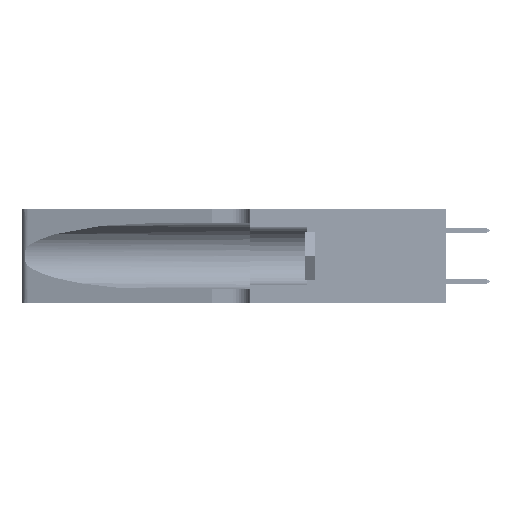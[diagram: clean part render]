
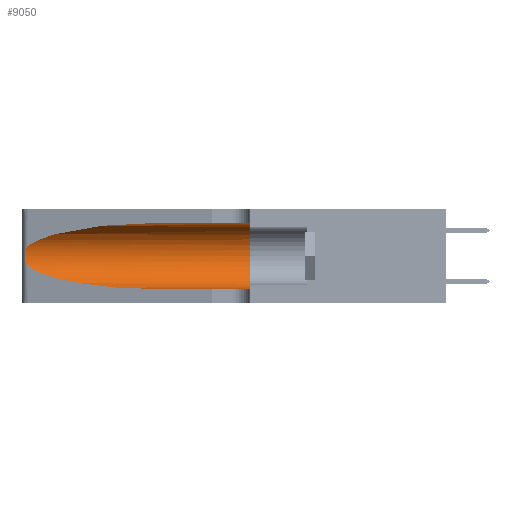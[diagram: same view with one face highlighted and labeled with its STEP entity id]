
A CAD part, left-side view. The second image highlights one B-rep face of the part: STEP entity #9050.
In plain terms, the highlighted cylindrical face has radius 3.308 mm (diameter 6.617 mm), a partial arc.
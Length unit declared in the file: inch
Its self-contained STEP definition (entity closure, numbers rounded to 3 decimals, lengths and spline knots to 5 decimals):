
#23 = VERTEX_POINT ( 'NONE', #31470 ) ;
#273 = CARTESIAN_POINT ( 'NONE',  ( 0.26075, 1.23896, 0.19203 ) ) ;
#2504 = CARTESIAN_POINT ( 'NONE',  ( 0.1305, 1.61858, 0.185 ) ) ;
#2601 = VERTEX_POINT ( 'NONE', #44118 ) ;
#2949 = CARTESIAN_POINT ( 'NONE',  ( 0.1305, 0.35, 0.185 ) ) ;
#3260 = AXIS2_PLACEMENT_3D ( 'NONE', #2504, #6538, #38540 ) ;
#3950 = CARTESIAN_POINT ( 'NONE',  ( 0.25787, 1.23484, 0.2124 ) ) ;
#6538 = DIRECTION ( 'NONE',  ( 0., -1., 0. ) ) ;
#7451 = CYLINDRICAL_SURFACE ( 'NONE', #3260, 0.13025 ) ;
#7989 = CIRCLE ( 'NONE', #35753, 0.13025 ) ;
#8011 = CARTESIAN_POINT ( 'NONE',  ( 0.1305, 1.61858, 0.31525 ) ) ;
#9050 = ADVANCED_FACE ( 'NONE', ( #36763 ), #7451, .F. ) ;
#10402 = DIRECTION ( 'NONE',  ( 0., -1., 0. ) ) ;
#10973 = DIRECTION ( 'NONE',  ( 0., 0., 1. ) ) ;
#11427 = CARTESIAN_POINT ( 'NONE',  ( 0.2373, 1.15595, 0.08982 ) ) ;
#11618 = CARTESIAN_POINT ( 'NONE',  ( 0.25639, 1.23186, 0.15144 ) ) ;
#13715 = EDGE_CURVE ( 'NONE', #27777, #23, #7989, .T. ) ;
#14352 = VERTEX_POINT ( 'NONE', #33731 ) ;
#14677 = CARTESIAN_POINT ( 'NONE',  ( 0.2373, 1.15595, 0.28018 ) ) ;
#16344 = LINE ( 'NONE', #8011, #45632 ) ;
#19237 = CARTESIAN_POINT ( 'NONE',  ( 0.18966, 0.96281, 0.05475 ) ) ;
#19596 = CARTESIAN_POINT ( 'NONE',  ( 0.25856, 1.23593, 0.16098 ) ) ;
#21000 = ORIENTED_EDGE ( 'NONE', *, *, #13715, .F. ) ;
#22015 = ORIENTED_EDGE ( 'NONE', *, *, #41227, .T. ) ;
#22273 = DIRECTION ( 'NONE',  ( 0., 1., 0. ) ) ;
#22543 = VERTEX_POINT ( 'NONE', #26861 ) ;
#23391 = CARTESIAN_POINT ( 'NONE',  ( 0.25487, 1.22718, 0.14631 ) ) ;
#24640 = EDGE_CURVE ( 'NONE', #2601, #14352, #43878, .T. ) ;
#24717 = VERTEX_POINT ( 'NONE', #51259 ) ;
#25894 = ORIENTED_EDGE ( 'NONE', *, *, #34208, .F. ) ;
#26861 = CARTESIAN_POINT ( 'NONE',  ( 0.1305, 0.72297, 0.05475 ) ) ;
#26908 = EDGE_CURVE ( 'NONE', #14352, #24717, #39383, .T. ) ;
#27451 = CARTESIAN_POINT ( 'NONE',  ( 0.25555, 1.22994, 0.2215 ) ) ;
#27771 = CARTESIAN_POINT ( 'NONE',  ( 0.25639, 1.23184, 0.21858 ) ) ;
#27777 = VERTEX_POINT ( 'NONE', #49011 ) ;
#28128 = CARTESIAN_POINT ( 'NONE',  ( 0.25854, 1.2359, 0.20912 ) ) ;
#28505 =( BOUNDED_CURVE ( )  B_SPLINE_CURVE ( 3, ( #23391, #11427, #19237, #46814 ),
 .UNSPECIFIED., .F., .F. ) 
 B_SPLINE_CURVE_WITH_KNOTS ( ( 4, 4 ),
 ( 3.44316, 4.71239 ),
 .UNSPECIFIED. ) 
 CURVE ( )  GEOMETRIC_REPRESENTATION_ITEM ( )  RATIONAL_B_SPLINE_CURVE ( ( 1., 0.87, 0.87, 1. ) ) 
 REPRESENTATION_ITEM ( '' )  );
#30803 = VECTOR ( 'NONE', #10402, 39.37008 ) ;
#31297 = CARTESIAN_POINT ( 'NONE',  ( 0.26018, 1.23835, 0.19895 ) ) ;
#31470 = CARTESIAN_POINT ( 'NONE',  ( 0.1305, 0.35, 0.05475 ) ) ;
#31965 = CARTESIAN_POINT ( 'NONE',  ( 0.25555, 1.22993, 0.14849 ) ) ;
#32906 = ORIENTED_EDGE ( 'NONE', *, *, #35516, .T. ) ;
#33531 = EDGE_LOOP ( 'NONE', ( #41309, #37654, #32906, #22015, #21000, #25894 ) ) ;
#33731 = CARTESIAN_POINT ( 'NONE',  ( 0.25487, 1.22718, 0.22369 ) ) ;
#34208 = EDGE_CURVE ( 'NONE', #2601, #27777, #16344, .T. ) ;
#34260 = CARTESIAN_POINT ( 'NONE',  ( 0.1305, 1.61858, 0.05475 ) ) ;
#35516 = EDGE_CURVE ( 'NONE', #24717, #22543, #28505, .T. ) ;
#35753 = AXIS2_PLACEMENT_3D ( 'NONE', #2949, #22273, #10973 ) ;
#36763 = FACE_OUTER_BOUND ( 'NONE', #33531, .T. ) ;
#37636 = LINE ( 'NONE', #34260, #30803 ) ;
#37654 = ORIENTED_EDGE ( 'NONE', *, *, #26908, .T. ) ;
#38328 = CARTESIAN_POINT ( 'NONE',  ( 0.18966, 0.96281, 0.31525 ) ) ;
#38540 = DIRECTION ( 'NONE',  ( 0., 0., -1. ) ) ;
#39309 = CARTESIAN_POINT ( 'NONE',  ( 0.26075, 1.23896, 0.178 ) ) ;
#39383 = B_SPLINE_CURVE_WITH_KNOTS ( 'NONE', 3,
 ( #43495, #27451, #27771, #3950, #28128, #31297, #273, #39309, #44000, #19596, #39822, #11618, #31965, #39479 ),
 .UNSPECIFIED., .F., .F.,
 ( 4, 2, 2, 2, 2, 2, 4 ),
 ( 0., 0.00027, 0.00053, 0.00107, 0.0016, 0.00187, 0.00214 ),
 .UNSPECIFIED. ) ;
#39479 = CARTESIAN_POINT ( 'NONE',  ( 0.25487, 1.22718, 0.14631 ) ) ;
#39822 = CARTESIAN_POINT ( 'NONE',  ( 0.25789, 1.23486, 0.15765 ) ) ;
#41227 = EDGE_CURVE ( 'NONE', #22543, #23, #37636, .T. ) ;
#41309 = ORIENTED_EDGE ( 'NONE', *, *, #24640, .T. ) ;
#43495 = CARTESIAN_POINT ( 'NONE',  ( 0.25487, 1.22718, 0.22369 ) ) ;
#43878 =( BOUNDED_CURVE ( )  B_SPLINE_CURVE ( 3, ( #50253, #38328, #14677, #46542 ),
 .UNSPECIFIED., .F., .F. ) 
 B_SPLINE_CURVE_WITH_KNOTS ( ( 4, 4 ),
 ( 1.5708, 2.84003 ),
 .UNSPECIFIED. ) 
 CURVE ( )  GEOMETRIC_REPRESENTATION_ITEM ( )  RATIONAL_B_SPLINE_CURVE ( ( 1., 0.87, 0.87, 1. ) ) 
 REPRESENTATION_ITEM ( '' )  );
#44000 = CARTESIAN_POINT ( 'NONE',  ( 0.26017, 1.23833, 0.17102 ) ) ;
#44118 = CARTESIAN_POINT ( 'NONE',  ( 0.1305, 0.72297, 0.31525 ) ) ;
#45632 = VECTOR ( 'NONE', #47929, 39.37008 ) ;
#46542 = CARTESIAN_POINT ( 'NONE',  ( 0.25487, 1.22718, 0.22369 ) ) ;
#46814 = CARTESIAN_POINT ( 'NONE',  ( 0.1305, 0.72297, 0.05475 ) ) ;
#47929 = DIRECTION ( 'NONE',  ( 0., -1., 0. ) ) ;
#49011 = CARTESIAN_POINT ( 'NONE',  ( 0.1305, 0.35, 0.31525 ) ) ;
#50253 = CARTESIAN_POINT ( 'NONE',  ( 0.1305, 0.72297, 0.31525 ) ) ;
#51259 = CARTESIAN_POINT ( 'NONE',  ( 0.25487, 1.22718, 0.14631 ) ) ;
